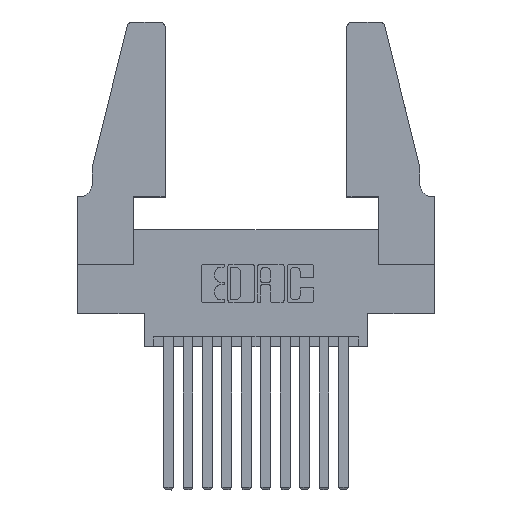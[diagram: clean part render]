
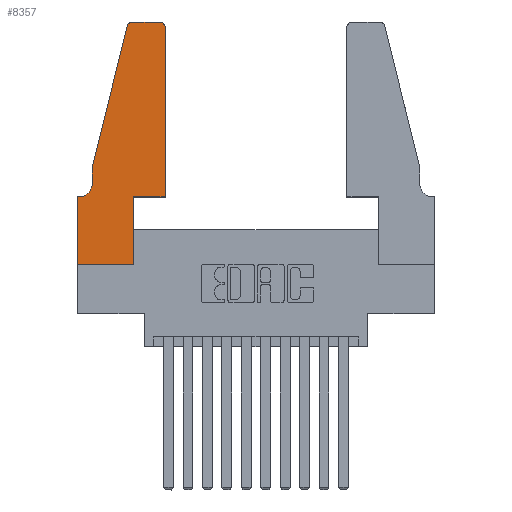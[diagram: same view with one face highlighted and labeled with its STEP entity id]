
A CAD part, top view. The second image highlights one B-rep face of the part: STEP entity #8357.
In plain terms, the highlighted planar face has unit normal (0, 0, 1).
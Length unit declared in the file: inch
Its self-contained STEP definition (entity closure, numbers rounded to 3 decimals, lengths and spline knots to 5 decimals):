
#19 = FACE_OUTER_BOUND ( 'NONE', #12496, .T. ) ;
#22 = VECTOR ( 'NONE', #6745, 39.37008 ) ;
#63 = EDGE_CURVE ( 'NONE', #8864, #465, #714, .T. ) ;
#465 = VERTEX_POINT ( 'NONE', #5147 ) ;
#531 = DIRECTION ( 'NONE',  ( 0., 0., 1. ) ) ;
#664 = CARTESIAN_POINT ( 'NONE',  ( 0.284, 1.22, 0.37 ) ) ;
#714 = LINE ( 'NONE', #4405, #22 ) ;
#761 = DIRECTION ( 'NONE',  ( 0., 0., 1. ) ) ;
#863 = CARTESIAN_POINT ( 'NONE',  ( 0.0755, 0.5, 0.37 ) ) ;
#1268 = DIRECTION ( 'NONE',  ( 0., -1., 0. ) ) ;
#1487 = DIRECTION ( 'NONE',  ( -1., 0., 0. ) ) ;
#1721 = EDGE_CURVE ( 'NONE', #8254, #5655, #5020, .T. ) ;
#1792 = CARTESIAN_POINT ( 'NONE',  ( 0.4205, 1.22, 0.37 ) ) ;
#1920 = VERTEX_POINT ( 'NONE', #6239 ) ;
#2078 = VECTOR ( 'NONE', #8125, 39.37008 ) ;
#2132 = VERTEX_POINT ( 'NONE', #2207 ) ;
#2207 = CARTESIAN_POINT ( 'NONE',  ( 0.25487, 1.22718, 0.37 ) ) ;
#2252 = CIRCLE ( 'NONE', #5825, 0.07 ) ;
#2323 = ORIENTED_EDGE ( 'NONE', *, *, #6471, .T. ) ;
#2549 = CARTESIAN_POINT ( 'NONE',  ( 0.0055, 0.35, 0.37 ) ) ;
#2927 = EDGE_CURVE ( 'NONE', #7503, #1920, #13591, .T. ) ;
#3128 = LINE ( 'NONE', #5659, #10685 ) ;
#3153 = EDGE_CURVE ( 'NONE', #5655, #2132, #4843, .T. ) ;
#3175 = ORIENTED_EDGE ( 'NONE', *, *, #2927, .T. ) ;
#3234 = LINE ( 'NONE', #863, #9571 ) ;
#3258 = VECTOR ( 'NONE', #5150, 39.37008 ) ;
#3323 = AXIS2_PLACEMENT_3D ( 'NONE', #12742, #531, #6058 ) ;
#3909 = VECTOR ( 'NONE', #13232, 39.37008 ) ;
#4215 = CARTESIAN_POINT ( 'NONE',  ( 0.284, 1.25, 0.37 ) ) ;
#4405 = CARTESIAN_POINT ( 'NONE',  ( 0.4505, 0.35, 0.37 ) ) ;
#4445 = EDGE_CURVE ( 'NONE', #4537, #5274, #3234, .T. ) ;
#4537 = VERTEX_POINT ( 'NONE', #10793 ) ;
#4546 = CARTESIAN_POINT ( 'NONE',  ( 0.4205, 1.25, 0.37 ) ) ;
#4615 = CARTESIAN_POINT ( 'NONE',  ( 0.2865, 0., 0.37 ) ) ;
#4800 = CARTESIAN_POINT ( 'NONE',  ( 0.2865, 0.35, 0.37 ) ) ;
#4843 = CIRCLE ( 'NONE', #5646, 0.03 ) ;
#5020 = LINE ( 'NONE', #11434, #2078 ) ;
#5127 = DIRECTION ( 'NONE',  ( 0., 0., 1. ) ) ;
#5147 = CARTESIAN_POINT ( 'NONE',  ( 0.4505, 0.35, 0.37 ) ) ;
#5150 = DIRECTION ( 'NONE',  ( 1., 0., 0. ) ) ;
#5274 = VERTEX_POINT ( 'NONE', #8096 ) ;
#5493 = AXIS2_PLACEMENT_3D ( 'NONE', #1792, #5127, #14116 ) ;
#5532 = LINE ( 'NONE', #14101, #11401 ) ;
#5646 = AXIS2_PLACEMENT_3D ( 'NONE', #664, #761, #8449 ) ;
#5655 = VERTEX_POINT ( 'NONE', #4215 ) ;
#5659 = CARTESIAN_POINT ( 'NONE',  ( 0.0755, 0.35, 0.37 ) ) ;
#5727 = ORIENTED_EDGE ( 'NONE', *, *, #9433, .T. ) ;
#5781 = ORIENTED_EDGE ( 'NONE', *, *, #7524, .T. ) ;
#5825 = AXIS2_PLACEMENT_3D ( 'NONE', #8057, #13405, #1487 ) ;
#6058 = DIRECTION ( 'NONE',  ( 1., 0., 0. ) ) ;
#6203 = EDGE_CURVE ( 'NONE', #2132, #4537, #12702, .T. ) ;
#6239 = CARTESIAN_POINT ( 'NONE',  ( 0., 0., 0.37 ) ) ;
#6471 = EDGE_CURVE ( 'NONE', #10243, #8864, #9915, .T. ) ;
#6540 = LINE ( 'NONE', #9855, #3258 ) ;
#6745 = DIRECTION ( 'NONE',  ( 1., 0., 0. ) ) ;
#7010 = DIRECTION ( 'NONE',  ( 0., 1., 0. ) ) ;
#7173 = PLANE ( 'NONE',  #3323 ) ;
#7373 = VERTEX_POINT ( 'NONE', #13910 ) ;
#7503 = VERTEX_POINT ( 'NONE', #10837 ) ;
#7524 = EDGE_CURVE ( 'NONE', #7373, #8254, #11271, .T. ) ;
#7706 = CARTESIAN_POINT ( 'NONE',  ( 0., 0., 0.37 ) ) ;
#8057 = CARTESIAN_POINT ( 'NONE',  ( 0.0055, 0.42, 0.37 ) ) ;
#8096 = CARTESIAN_POINT ( 'NONE',  ( 0.0755, 0.42, 0.37 ) ) ;
#8125 = DIRECTION ( 'NONE',  ( -1., 0., 0. ) ) ;
#8254 = VERTEX_POINT ( 'NONE', #4546 ) ;
#8357 = ADVANCED_FACE ( 'NONE', ( #19 ), #7173, .T. ) ;
#8449 = DIRECTION ( 'NONE',  ( 1., 0., 0. ) ) ;
#8864 = VERTEX_POINT ( 'NONE', #11713 ) ;
#8998 = EDGE_CURVE ( 'NONE', #465, #7373, #5532, .T. ) ;
#9071 = ORIENTED_EDGE ( 'NONE', *, *, #13344, .T. ) ;
#9433 = EDGE_CURVE ( 'NONE', #14011, #7503, #3128, .T. ) ;
#9571 = VECTOR ( 'NONE', #12925, 39.37008 ) ;
#9855 = CARTESIAN_POINT ( 'NONE',  ( 0., 0., 0.37 ) ) ;
#9915 = LINE ( 'NONE', #4800, #10611 ) ;
#10195 = ORIENTED_EDGE ( 'NONE', *, *, #3153, .T. ) ;
#10243 = VERTEX_POINT ( 'NONE', #4615 ) ;
#10611 = VECTOR ( 'NONE', #7010, 39.37008 ) ;
#10629 = ORIENTED_EDGE ( 'NONE', *, *, #8998, .T. ) ;
#10685 = VECTOR ( 'NONE', #13347, 39.37008 ) ;
#10752 = ORIENTED_EDGE ( 'NONE', *, *, #1721, .T. ) ;
#10793 = CARTESIAN_POINT ( 'NONE',  ( 0.0755, 0.5, 0.37 ) ) ;
#10837 = CARTESIAN_POINT ( 'NONE',  ( 0., 0.35, 0.37 ) ) ;
#10986 = CARTESIAN_POINT ( 'NONE',  ( 0.0755, 0.5, 0.37 ) ) ;
#11174 = VECTOR ( 'NONE', #1268, 39.37008 ) ;
#11271 = CIRCLE ( 'NONE', #5493, 0.03 ) ;
#11386 = ORIENTED_EDGE ( 'NONE', *, *, #63, .T. ) ;
#11401 = VECTOR ( 'NONE', #11922, 39.37008 ) ;
#11434 = CARTESIAN_POINT ( 'NONE',  ( 0.2605, 1.25, 0.37 ) ) ;
#11510 = ORIENTED_EDGE ( 'NONE', *, *, #12173, .T. ) ;
#11713 = CARTESIAN_POINT ( 'NONE',  ( 0.2865, 0.35, 0.37 ) ) ;
#11922 = DIRECTION ( 'NONE',  ( 0., 1., 0. ) ) ;
#12173 = EDGE_CURVE ( 'NONE', #5274, #14011, #2252, .T. ) ;
#12496 = EDGE_LOOP ( 'NONE', ( #10752, #10195, #12761, #13693, #11510, #5727, #3175, #9071, #2323, #11386, #10629, #5781 ) ) ;
#12702 = LINE ( 'NONE', #10986, #3909 ) ;
#12742 = CARTESIAN_POINT ( 'NONE',  ( 0., 0.35, 0.37 ) ) ;
#12761 = ORIENTED_EDGE ( 'NONE', *, *, #6203, .T. ) ;
#12925 = DIRECTION ( 'NONE',  ( 0., -1., 0. ) ) ;
#13232 = DIRECTION ( 'NONE',  ( -0.239, -0.971, 0. ) ) ;
#13344 = EDGE_CURVE ( 'NONE', #1920, #10243, #6540, .T. ) ;
#13347 = DIRECTION ( 'NONE',  ( -1., 0., 0. ) ) ;
#13405 = DIRECTION ( 'NONE',  ( 0., 0., -1. ) ) ;
#13591 = LINE ( 'NONE', #7706, #11174 ) ;
#13693 = ORIENTED_EDGE ( 'NONE', *, *, #4445, .T. ) ;
#13910 = CARTESIAN_POINT ( 'NONE',  ( 0.4505, 1.22, 0.37 ) ) ;
#14011 = VERTEX_POINT ( 'NONE', #2549 ) ;
#14101 = CARTESIAN_POINT ( 'NONE',  ( 0.4505, 0.35, 0.37 ) ) ;
#14116 = DIRECTION ( 'NONE',  ( 1., 0., 0. ) ) ;
